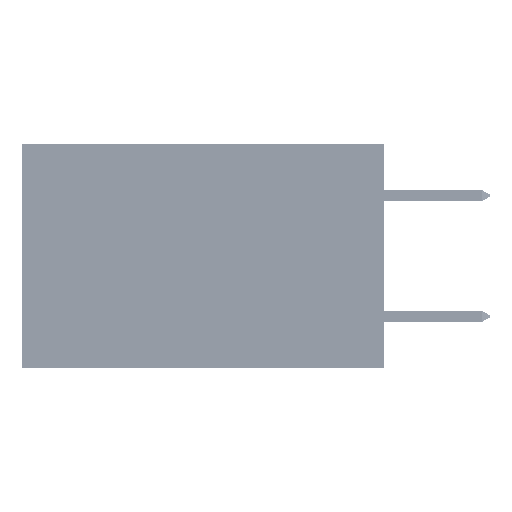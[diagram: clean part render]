
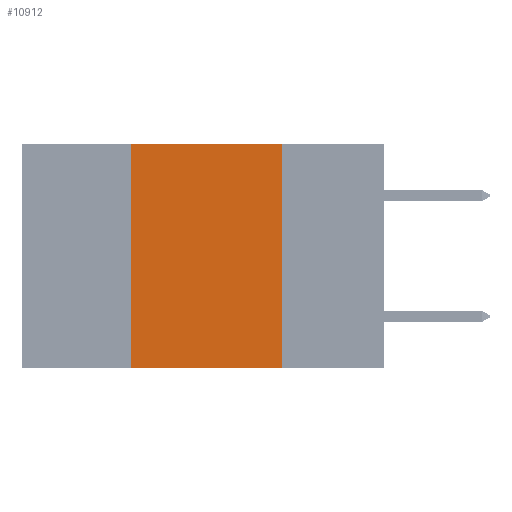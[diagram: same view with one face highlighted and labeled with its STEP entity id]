
A CAD part, left-side view. The second image highlights one B-rep face of the part: STEP entity #10912.
In plain terms, the highlighted planar face has unit normal (-1, 0, 0).
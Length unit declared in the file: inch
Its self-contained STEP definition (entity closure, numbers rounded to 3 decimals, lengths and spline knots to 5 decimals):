
#2520 = LINE ( 'NONE', #12722, #42235 ) ;
#5661 = DIRECTION ( 'NONE',  ( 0., -1., 0. ) ) ;
#7722 = EDGE_LOOP ( 'NONE', ( #24994, #21194, #14545, #19322 ) ) ;
#8505 = EDGE_CURVE ( 'NONE', #17132, #41969, #11557, .T. ) ;
#8984 = DIRECTION ( 'NONE',  ( 0., -1., 0. ) ) ;
#10912 = ADVANCED_FACE ( 'NONE', ( #21144 ), #26512, .F. ) ;
#10984 = DIRECTION ( 'NONE',  ( 1., 0., 0. ) ) ;
#11557 = LINE ( 'NONE', #25172, #15813 ) ;
#12722 = CARTESIAN_POINT ( 'NONE',  ( 0., 0.6, 0. ) ) ;
#13131 = EDGE_CURVE ( 'NONE', #47831, #17132, #2520, .T. ) ;
#14545 = ORIENTED_EDGE ( 'NONE', *, *, #43451, .F. ) ;
#15813 = VECTOR ( 'NONE', #45291, 39.37008 ) ;
#17132 = VERTEX_POINT ( 'NONE', #22606 ) ;
#17641 = EDGE_CURVE ( 'NONE', #49800, #41969, #20479, .T. ) ;
#19322 = ORIENTED_EDGE ( 'NONE', *, *, #17641, .T. ) ;
#20479 = LINE ( 'NONE', #28674, #50406 ) ;
#21144 = FACE_OUTER_BOUND ( 'NONE', #7722, .T. ) ;
#21194 = ORIENTED_EDGE ( 'NONE', *, *, #13131, .F. ) ;
#22548 = AXIS2_PLACEMENT_3D ( 'NONE', #26348, #10984, #38455 ) ;
#22606 = CARTESIAN_POINT ( 'NONE',  ( 0., 0.17, 0. ) ) ;
#24994 = ORIENTED_EDGE ( 'NONE', *, *, #8505, .F. ) ;
#25061 = DIRECTION ( 'NONE',  ( 0., 0., 1. ) ) ;
#25172 = CARTESIAN_POINT ( 'NONE',  ( 0., 0.17, 0. ) ) ;
#26348 = CARTESIAN_POINT ( 'NONE',  ( 0., 0.6, 0. ) ) ;
#26512 = PLANE ( 'NONE',  #22548 ) ;
#28674 = CARTESIAN_POINT ( 'NONE',  ( 0., 0.6, -0.37 ) ) ;
#32876 = VECTOR ( 'NONE', #25061, 39.37008 ) ;
#35289 = CARTESIAN_POINT ( 'NONE',  ( 0., 0.17, -0.37 ) ) ;
#38029 = CARTESIAN_POINT ( 'NONE',  ( 0., 0.42, 0. ) ) ;
#38455 = DIRECTION ( 'NONE',  ( 0., 0., -1. ) ) ;
#38937 = CARTESIAN_POINT ( 'NONE',  ( 0., 0.42, -0.37 ) ) ;
#41969 = VERTEX_POINT ( 'NONE', #35289 ) ;
#42235 = VECTOR ( 'NONE', #8984, 39.37008 ) ;
#43451 = EDGE_CURVE ( 'NONE', #49800, #47831, #49995, .T. ) ;
#45291 = DIRECTION ( 'NONE',  ( 0., 0., -1. ) ) ;
#47831 = VERTEX_POINT ( 'NONE', #38029 ) ;
#48941 = CARTESIAN_POINT ( 'NONE',  ( 0., 0.42, 0. ) ) ;
#49800 = VERTEX_POINT ( 'NONE', #38937 ) ;
#49995 = LINE ( 'NONE', #48941, #32876 ) ;
#50406 = VECTOR ( 'NONE', #5661, 39.37008 ) ;
